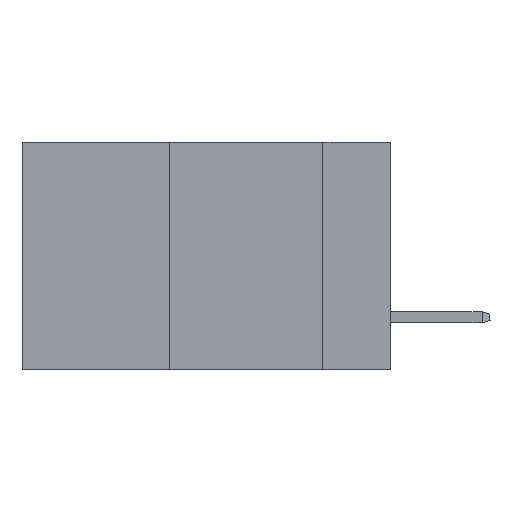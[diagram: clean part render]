
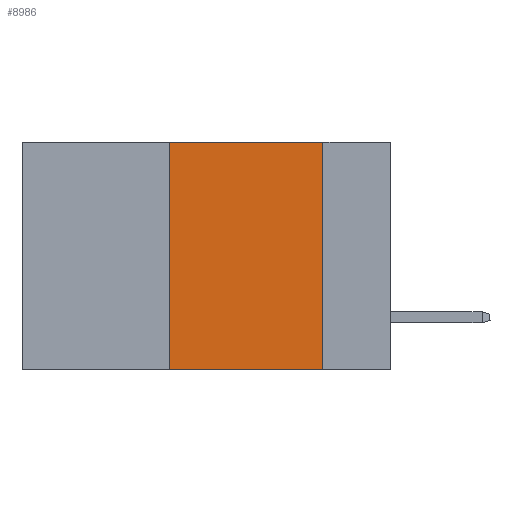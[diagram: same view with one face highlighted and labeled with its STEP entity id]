
A CAD part, left-side view. The second image highlights one B-rep face of the part: STEP entity #8986.
In plain terms, the highlighted planar face has unit normal (-1, 0, 0).
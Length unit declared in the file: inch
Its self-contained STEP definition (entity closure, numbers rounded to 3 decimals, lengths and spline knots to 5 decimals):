
#200 = CARTESIAN_POINT ( 'NONE',  ( 0., 0.6, -0.37 ) ) ;
#345 = ORIENTED_EDGE ( 'NONE', *, *, #16884, .T. ) ;
#931 = PLANE ( 'NONE',  #13750 ) ;
#1379 = CARTESIAN_POINT ( 'NONE',  ( 0., 0.36, 0. ) ) ;
#1610 = ORIENTED_EDGE ( 'NONE', *, *, #4271, .F. ) ;
#2107 = VERTEX_POINT ( 'NONE', #6966 ) ;
#2189 = VECTOR ( 'NONE', #9670, 39.37008 ) ;
#2260 = DIRECTION ( 'NONE',  ( 0., 0., -1. ) ) ;
#3002 = EDGE_LOOP ( 'NONE', ( #1610, #17430, #15066, #345 ) ) ;
#3095 = FACE_OUTER_BOUND ( 'NONE', #3002, .T. ) ;
#3544 = LINE ( 'NONE', #1379, #5673 ) ;
#4271 = EDGE_CURVE ( 'NONE', #10717, #10544, #5795, .T. ) ;
#5673 = VECTOR ( 'NONE', #9339, 39.37008 ) ;
#5750 = DIRECTION ( 'NONE',  ( 0., -1., 0. ) ) ;
#5795 = LINE ( 'NONE', #11095, #2189 ) ;
#6160 = CARTESIAN_POINT ( 'NONE',  ( 0., 0.36, 0. ) ) ;
#6966 = CARTESIAN_POINT ( 'NONE',  ( 0., 0.36, -0.37 ) ) ;
#7725 = DIRECTION ( 'NONE',  ( 0., -1., 0. ) ) ;
#8889 = CARTESIAN_POINT ( 'NONE',  ( 0., 0.11, -0.37 ) ) ;
#8986 = ADVANCED_FACE ( 'NONE', ( #3095 ), #931, .F. ) ;
#9339 = DIRECTION ( 'NONE',  ( 0., 0., 1. ) ) ;
#9670 = DIRECTION ( 'NONE',  ( 0., 0., -1. ) ) ;
#10015 = VECTOR ( 'NONE', #5750, 39.37008 ) ;
#10412 = CARTESIAN_POINT ( 'NONE',  ( 0., 0.11, 0. ) ) ;
#10461 = CARTESIAN_POINT ( 'NONE',  ( 0., 0.6, 0. ) ) ;
#10544 = VERTEX_POINT ( 'NONE', #8889 ) ;
#10642 = EDGE_CURVE ( 'NONE', #11807, #10717, #14744, .T. ) ;
#10717 = VERTEX_POINT ( 'NONE', #10412 ) ;
#11095 = CARTESIAN_POINT ( 'NONE',  ( 0., 0.11, 0. ) ) ;
#11807 = VERTEX_POINT ( 'NONE', #6160 ) ;
#12163 = CARTESIAN_POINT ( 'NONE',  ( 0., 0.6, 0. ) ) ;
#12843 = VECTOR ( 'NONE', #7725, 39.37008 ) ;
#13247 = EDGE_CURVE ( 'NONE', #2107, #11807, #3544, .T. ) ;
#13750 = AXIS2_PLACEMENT_3D ( 'NONE', #10461, #15775, #2260 ) ;
#14744 = LINE ( 'NONE', #12163, #12843 ) ;
#15066 = ORIENTED_EDGE ( 'NONE', *, *, #13247, .F. ) ;
#15775 = DIRECTION ( 'NONE',  ( 1., 0., 0. ) ) ;
#15992 = LINE ( 'NONE', #200, #10015 ) ;
#16884 = EDGE_CURVE ( 'NONE', #2107, #10544, #15992, .T. ) ;
#17430 = ORIENTED_EDGE ( 'NONE', *, *, #10642, .F. ) ;
